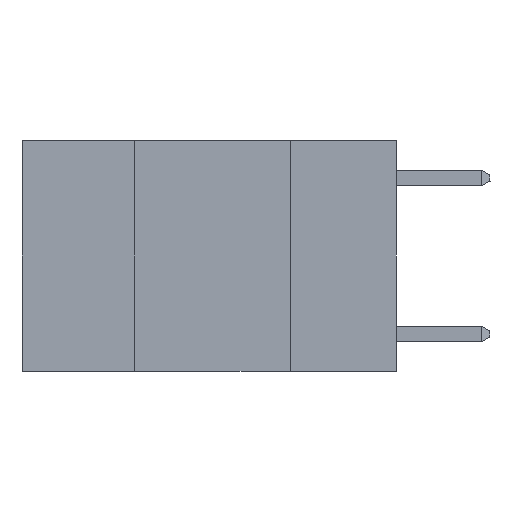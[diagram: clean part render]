
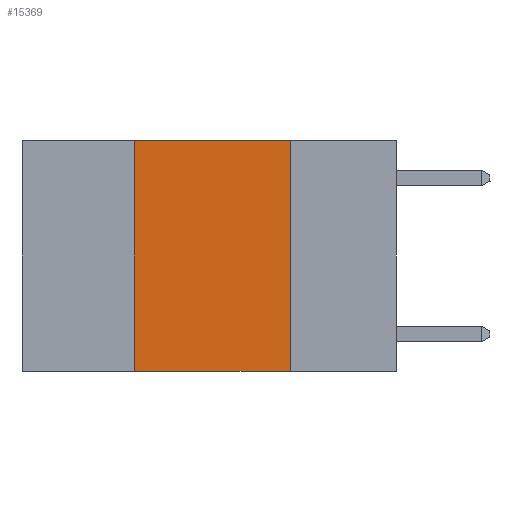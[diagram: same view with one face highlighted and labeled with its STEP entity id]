
A CAD part, left-side view. The second image highlights one B-rep face of the part: STEP entity #15369.
In plain terms, the highlighted planar face has unit normal (-1, 0, 0).
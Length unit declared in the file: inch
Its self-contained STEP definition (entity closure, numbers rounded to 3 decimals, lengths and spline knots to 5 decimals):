
#606 = DIRECTION ( 'NONE',  ( 1., 0., 0. ) ) ;
#1353 = EDGE_CURVE ( 'NONE', #5996, #2499, #1394, .T. ) ;
#1394 = LINE ( 'NONE', #6115, #1811 ) ;
#1413 = VERTEX_POINT ( 'NONE', #2800 ) ;
#1811 = VECTOR ( 'NONE', #8963, 39.37008 ) ;
#1976 = ORIENTED_EDGE ( 'NONE', *, *, #8128, .T. ) ;
#2499 = VERTEX_POINT ( 'NONE', #12872 ) ;
#2800 = CARTESIAN_POINT ( 'NONE',  ( 0., 0.17, 0. ) ) ;
#3138 = LINE ( 'NONE', #3775, #9299 ) ;
#3148 = ORIENTED_EDGE ( 'NONE', *, *, #8484, .F. ) ;
#3354 = EDGE_LOOP ( 'NONE', ( #3148, #5854, #4103, #1976 ) ) ;
#3748 = FACE_OUTER_BOUND ( 'NONE', #3354, .T. ) ;
#3775 = CARTESIAN_POINT ( 'NONE',  ( 0., 0.6, -0.37 ) ) ;
#4103 = ORIENTED_EDGE ( 'NONE', *, *, #1353, .F. ) ;
#5644 = PLANE ( 'NONE',  #7054 ) ;
#5854 = ORIENTED_EDGE ( 'NONE', *, *, #14424, .F. ) ;
#5996 = VERTEX_POINT ( 'NONE', #11558 ) ;
#6115 = CARTESIAN_POINT ( 'NONE',  ( 0., 0.42, 0. ) ) ;
#7054 = AXIS2_PLACEMENT_3D ( 'NONE', #9301, #606, #9356 ) ;
#7612 = LINE ( 'NONE', #13264, #13197 ) ;
#7896 = VECTOR ( 'NONE', #15087, 39.37008 ) ;
#8010 = CARTESIAN_POINT ( 'NONE',  ( 0., 0.17, 0. ) ) ;
#8128 = EDGE_CURVE ( 'NONE', #5996, #8453, #3138, .T. ) ;
#8453 = VERTEX_POINT ( 'NONE', #10456 ) ;
#8484 = EDGE_CURVE ( 'NONE', #1413, #8453, #13845, .T. ) ;
#8963 = DIRECTION ( 'NONE',  ( 0., 0., 1. ) ) ;
#9299 = VECTOR ( 'NONE', #11079, 39.37008 ) ;
#9301 = CARTESIAN_POINT ( 'NONE',  ( 0., 0.6, 0. ) ) ;
#9356 = DIRECTION ( 'NONE',  ( 0., 0., -1. ) ) ;
#10456 = CARTESIAN_POINT ( 'NONE',  ( 0., 0.17, -0.37 ) ) ;
#11079 = DIRECTION ( 'NONE',  ( 0., -1., 0. ) ) ;
#11558 = CARTESIAN_POINT ( 'NONE',  ( 0., 0.42, -0.37 ) ) ;
#12872 = CARTESIAN_POINT ( 'NONE',  ( 0., 0.42, 0. ) ) ;
#13197 = VECTOR ( 'NONE', #15550, 39.37008 ) ;
#13264 = CARTESIAN_POINT ( 'NONE',  ( 0., 0.6, 0. ) ) ;
#13845 = LINE ( 'NONE', #8010, #7896 ) ;
#14424 = EDGE_CURVE ( 'NONE', #2499, #1413, #7612, .T. ) ;
#15087 = DIRECTION ( 'NONE',  ( 0., 0., -1. ) ) ;
#15369 = ADVANCED_FACE ( 'NONE', ( #3748 ), #5644, .F. ) ;
#15550 = DIRECTION ( 'NONE',  ( 0., -1., 0. ) ) ;
